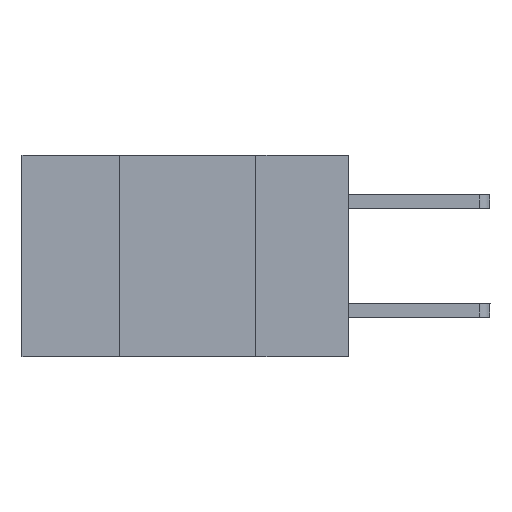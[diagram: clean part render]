
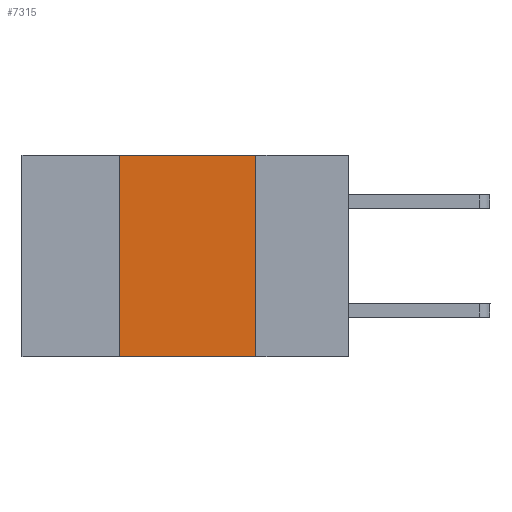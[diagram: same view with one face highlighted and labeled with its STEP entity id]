
A CAD part, left-side view. The second image highlights one B-rep face of the part: STEP entity #7315.
In plain terms, the highlighted planar face has unit normal (-1, 0, 0).
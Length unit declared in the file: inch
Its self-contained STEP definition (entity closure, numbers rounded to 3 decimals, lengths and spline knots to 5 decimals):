
#57 = VERTEX_POINT ( 'NONE', #4628 ) ;
#158 = DIRECTION ( 'NONE',  ( 0., -1., 0. ) ) ;
#1623 = ORIENTED_EDGE ( 'NONE', *, *, #9909, .T. ) ;
#1910 = LINE ( 'NONE', #6331, #2618 ) ;
#2618 = VECTOR ( 'NONE', #5662, 39.37008 ) ;
#2907 = EDGE_LOOP ( 'NONE', ( #8981, #3458, #8645, #1623 ) ) ;
#2983 = FACE_OUTER_BOUND ( 'NONE', #2907, .T. ) ;
#3066 = LINE ( 'NONE', #4853, #11192 ) ;
#3458 = ORIENTED_EDGE ( 'NONE', *, *, #4610, .F. ) ;
#3978 = EDGE_CURVE ( 'NONE', #8084, #5115, #1910, .T. ) ;
#4610 = EDGE_CURVE ( 'NONE', #7771, #8084, #9350, .T. ) ;
#4628 = CARTESIAN_POINT ( 'NONE',  ( 0., 0.42, -0.37 ) ) ;
#4698 = DIRECTION ( 'NONE',  ( 0., 0., 1. ) ) ;
#4853 = CARTESIAN_POINT ( 'NONE',  ( 0., 0.6, -0.37 ) ) ;
#5115 = VERTEX_POINT ( 'NONE', #7606 ) ;
#5370 = CARTESIAN_POINT ( 'NONE',  ( 0., 0.42, 0. ) ) ;
#5414 = CARTESIAN_POINT ( 'NONE',  ( 0., 0.6, 0. ) ) ;
#5555 = VECTOR ( 'NONE', #4698, 39.37008 ) ;
#5662 = DIRECTION ( 'NONE',  ( 0., 0., -1. ) ) ;
#5882 = DIRECTION ( 'NONE',  ( 0., -1., 0. ) ) ;
#6331 = CARTESIAN_POINT ( 'NONE',  ( 0., 0.17, 0. ) ) ;
#6425 = DIRECTION ( 'NONE',  ( 0., 0., -1. ) ) ;
#7010 = AXIS2_PLACEMENT_3D ( 'NONE', #9005, #7223, #6425 ) ;
#7036 = VECTOR ( 'NONE', #158, 39.37008 ) ;
#7223 = DIRECTION ( 'NONE',  ( 1., 0., 0. ) ) ;
#7315 = ADVANCED_FACE ( 'NONE', ( #2983 ), #8888, .F. ) ;
#7371 = EDGE_CURVE ( 'NONE', #57, #7771, #10156, .T. ) ;
#7606 = CARTESIAN_POINT ( 'NONE',  ( 0., 0.17, -0.37 ) ) ;
#7771 = VERTEX_POINT ( 'NONE', #5370 ) ;
#8084 = VERTEX_POINT ( 'NONE', #9561 ) ;
#8645 = ORIENTED_EDGE ( 'NONE', *, *, #7371, .F. ) ;
#8888 = PLANE ( 'NONE',  #7010 ) ;
#8981 = ORIENTED_EDGE ( 'NONE', *, *, #3978, .F. ) ;
#9005 = CARTESIAN_POINT ( 'NONE',  ( 0., 0.6, 0. ) ) ;
#9350 = LINE ( 'NONE', #5414, #7036 ) ;
#9561 = CARTESIAN_POINT ( 'NONE',  ( 0., 0.17, 0. ) ) ;
#9909 = EDGE_CURVE ( 'NONE', #57, #5115, #3066, .T. ) ;
#10156 = LINE ( 'NONE', #10623, #5555 ) ;
#10623 = CARTESIAN_POINT ( 'NONE',  ( 0., 0.42, 0. ) ) ;
#11192 = VECTOR ( 'NONE', #5882, 39.37008 ) ;
